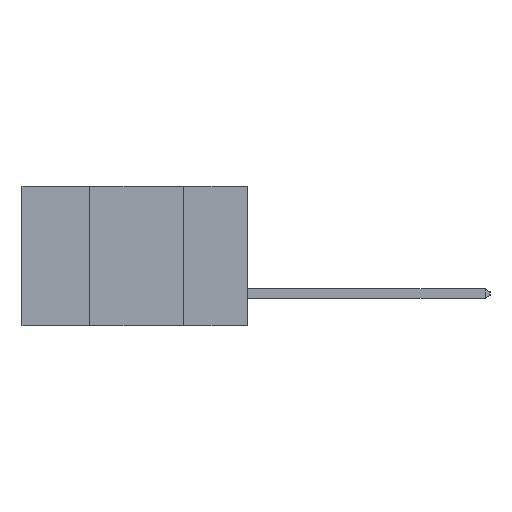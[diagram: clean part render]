
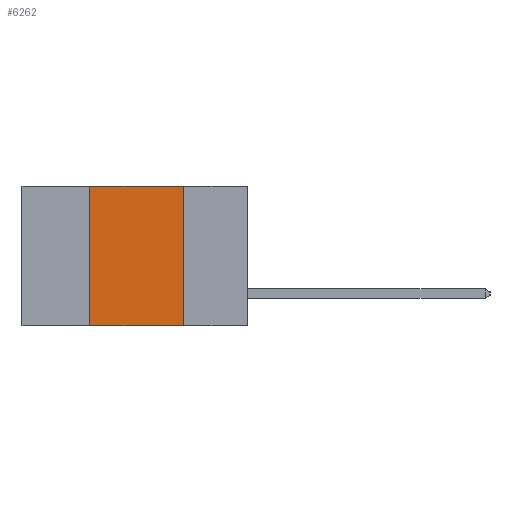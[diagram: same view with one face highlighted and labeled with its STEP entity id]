
A CAD part, left-side view. The second image highlights one B-rep face of the part: STEP entity #6262.
In plain terms, the highlighted planar face has unit normal (-1, 0, 0).
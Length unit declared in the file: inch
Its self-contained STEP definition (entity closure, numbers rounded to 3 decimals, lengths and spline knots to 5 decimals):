
#31 = CARTESIAN_POINT ( 'NONE',  ( 0., 0.17, 0. ) ) ;
#481 = CARTESIAN_POINT ( 'NONE',  ( 0., 0.6, 0. ) ) ;
#606 = CARTESIAN_POINT ( 'NONE',  ( 0., 0.17, -0.37 ) ) ;
#1449 = EDGE_CURVE ( 'NONE', #2643, #9302, #11746, .T. ) ;
#2391 = DIRECTION ( 'NONE',  ( 0., -1., 0. ) ) ;
#2643 = VERTEX_POINT ( 'NONE', #14026 ) ;
#2712 = CARTESIAN_POINT ( 'NONE',  ( 0., 0.6, 0. ) ) ;
#2872 = VECTOR ( 'NONE', #7879, 39.37008 ) ;
#2880 = ORIENTED_EDGE ( 'NONE', *, *, #13898, .T. ) ;
#2886 = DIRECTION ( 'NONE',  ( 0., 0., 1. ) ) ;
#2946 = VECTOR ( 'NONE', #6838, 39.37008 ) ;
#3019 = ORIENTED_EDGE ( 'NONE', *, *, #4198, .F. ) ;
#3361 = VECTOR ( 'NONE', #2886, 39.37008 ) ;
#4013 = EDGE_LOOP ( 'NONE', ( #4343, #5015, #3019, #2880 ) ) ;
#4198 = EDGE_CURVE ( 'NONE', #5936, #2643, #6384, .T. ) ;
#4343 = ORIENTED_EDGE ( 'NONE', *, *, #8712, .F. ) ;
#4647 = VERTEX_POINT ( 'NONE', #606 ) ;
#4822 = CARTESIAN_POINT ( 'NONE',  ( 0., 0.42, 0. ) ) ;
#5015 = ORIENTED_EDGE ( 'NONE', *, *, #1449, .F. ) ;
#5684 = CARTESIAN_POINT ( 'NONE',  ( 0., 0.6, -0.37 ) ) ;
#5936 = VERTEX_POINT ( 'NONE', #11232 ) ;
#6262 = ADVANCED_FACE ( 'NONE', ( #6877 ), #9006, .F. ) ;
#6384 = LINE ( 'NONE', #4822, #3361 ) ;
#6838 = DIRECTION ( 'NONE',  ( 0., -1., 0. ) ) ;
#6877 = FACE_OUTER_BOUND ( 'NONE', #4013, .T. ) ;
#7565 = AXIS2_PLACEMENT_3D ( 'NONE', #2712, #10233, #10116 ) ;
#7879 = DIRECTION ( 'NONE',  ( 0., 0., -1. ) ) ;
#7917 = CARTESIAN_POINT ( 'NONE',  ( 0., 0.17, 0. ) ) ;
#8712 = EDGE_CURVE ( 'NONE', #9302, #4647, #11730, .T. ) ;
#8908 = VECTOR ( 'NONE', #2391, 39.37008 ) ;
#9006 = PLANE ( 'NONE',  #7565 ) ;
#9302 = VERTEX_POINT ( 'NONE', #31 ) ;
#10116 = DIRECTION ( 'NONE',  ( 0., 0., -1. ) ) ;
#10233 = DIRECTION ( 'NONE',  ( 1., 0., 0. ) ) ;
#11232 = CARTESIAN_POINT ( 'NONE',  ( 0., 0.42, -0.37 ) ) ;
#11730 = LINE ( 'NONE', #7917, #2872 ) ;
#11746 = LINE ( 'NONE', #481, #8908 ) ;
#11796 = LINE ( 'NONE', #5684, #2946 ) ;
#13898 = EDGE_CURVE ( 'NONE', #5936, #4647, #11796, .T. ) ;
#14026 = CARTESIAN_POINT ( 'NONE',  ( 0., 0.42, 0. ) ) ;
